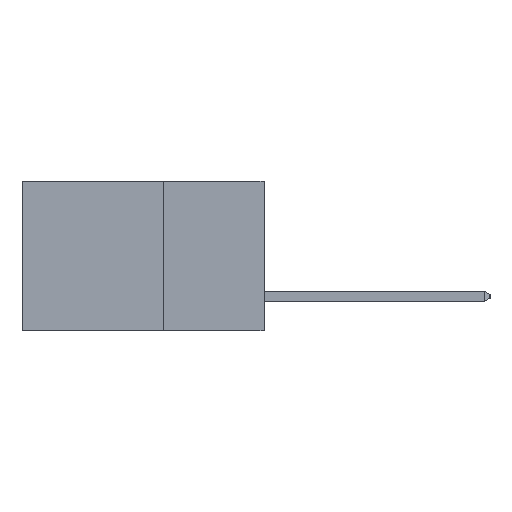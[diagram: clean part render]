
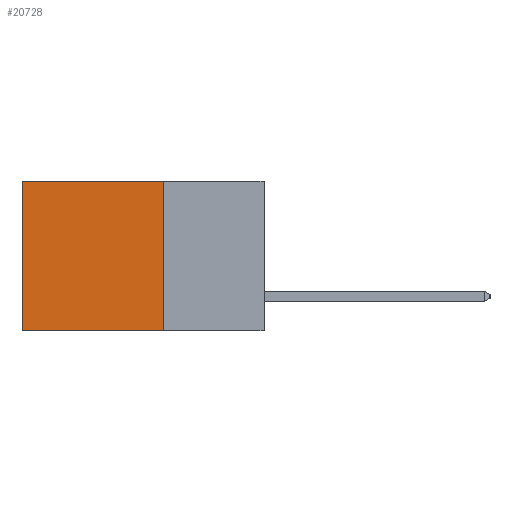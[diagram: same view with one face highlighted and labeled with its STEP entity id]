
A CAD part, left-side view. The second image highlights one B-rep face of the part: STEP entity #20728.
In plain terms, the highlighted planar face has unit normal (-1, 0, 0).
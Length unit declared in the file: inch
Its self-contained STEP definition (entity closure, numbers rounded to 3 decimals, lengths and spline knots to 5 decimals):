
#118 = LINE ( 'NONE', #15577, #18517 ) ;
#262 = CARTESIAN_POINT ( 'NONE',  ( 0.2615, 0.25, -0.37 ) ) ;
#2071 = DIRECTION ( 'NONE',  ( 0., 0., -1. ) ) ;
#2921 = CARTESIAN_POINT ( 'NONE',  ( 0.2615, 0.6, -0.37 ) ) ;
#3208 = LINE ( 'NONE', #14891, #7546 ) ;
#5076 = VERTEX_POINT ( 'NONE', #21026 ) ;
#5235 = EDGE_CURVE ( 'NONE', #19228, #5076, #18198, .T. ) ;
#7546 = VECTOR ( 'NONE', #14765, 39.37008 ) ;
#7620 = FACE_OUTER_BOUND ( 'NONE', #21550, .T. ) ;
#7738 = LINE ( 'NONE', #14652, #21130 ) ;
#7843 = EDGE_CURVE ( 'NONE', #5076, #12460, #118, .T. ) ;
#7907 = EDGE_CURVE ( 'NONE', #23036, #12460, #3208, .T. ) ;
#8581 = CARTESIAN_POINT ( 'NONE',  ( 0.2615, 0.25, 0. ) ) ;
#9918 = EDGE_CURVE ( 'NONE', #19228, #23036, #7738, .T. ) ;
#9919 = ORIENTED_EDGE ( 'NONE', *, *, #9918, .F. ) ;
#12460 = VERTEX_POINT ( 'NONE', #2921 ) ;
#13170 = DIRECTION ( 'NONE',  ( 1., 0., 0. ) ) ;
#14652 = CARTESIAN_POINT ( 'NONE',  ( 0.2615, 0.25, -0.37 ) ) ;
#14739 = DIRECTION ( 'NONE',  ( 0., 0., -1. ) ) ;
#14765 = DIRECTION ( 'NONE',  ( 0., 1., 0. ) ) ;
#14891 = CARTESIAN_POINT ( 'NONE',  ( 0.2615, 0.25, -0.37 ) ) ;
#15429 = DIRECTION ( 'NONE',  ( 0., 0., -1. ) ) ;
#15577 = CARTESIAN_POINT ( 'NONE',  ( 0.2615, 0.6, -0.37 ) ) ;
#16328 = CARTESIAN_POINT ( 'NONE',  ( 0.2615, 0.25, -0.37 ) ) ;
#16668 = PLANE ( 'NONE',  #17408 ) ;
#16787 = DIRECTION ( 'NONE',  ( 0., 1., 0. ) ) ;
#16895 = CARTESIAN_POINT ( 'NONE',  ( 0.2615, 0.25, 0. ) ) ;
#17408 = AXIS2_PLACEMENT_3D ( 'NONE', #262, #13170, #2071 ) ;
#17642 = ORIENTED_EDGE ( 'NONE', *, *, #7907, .F. ) ;
#17892 = ORIENTED_EDGE ( 'NONE', *, *, #7843, .T. ) ;
#18198 = LINE ( 'NONE', #16895, #21736 ) ;
#18517 = VECTOR ( 'NONE', #15429, 39.37008 ) ;
#19228 = VERTEX_POINT ( 'NONE', #8581 ) ;
#20728 = ADVANCED_FACE ( 'NONE', ( #7620 ), #16668, .F. ) ;
#21000 = ORIENTED_EDGE ( 'NONE', *, *, #5235, .T. ) ;
#21026 = CARTESIAN_POINT ( 'NONE',  ( 0.2615, 0.6, 0. ) ) ;
#21130 = VECTOR ( 'NONE', #14739, 39.37008 ) ;
#21550 = EDGE_LOOP ( 'NONE', ( #17892, #17642, #9919, #21000 ) ) ;
#21736 = VECTOR ( 'NONE', #16787, 39.37008 ) ;
#23036 = VERTEX_POINT ( 'NONE', #16328 ) ;
